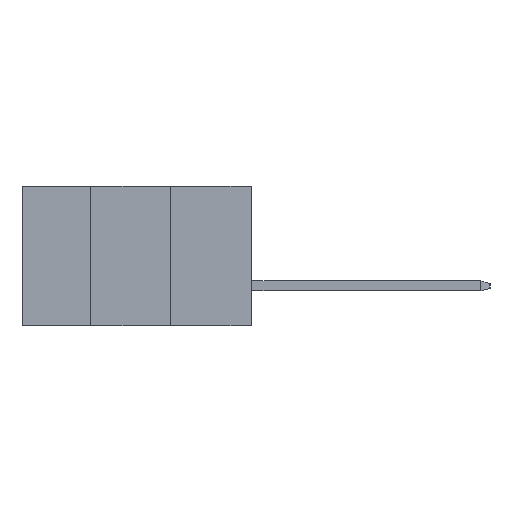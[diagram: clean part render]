
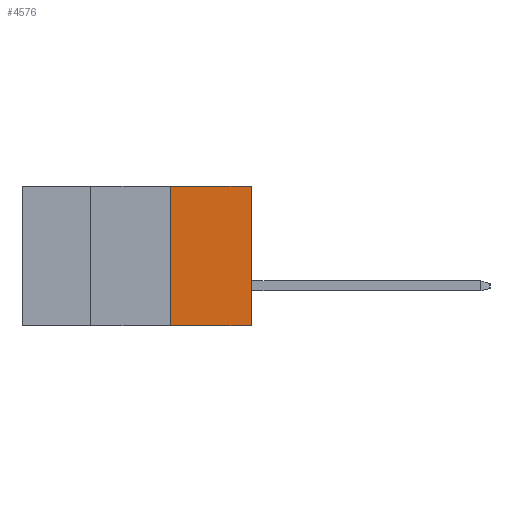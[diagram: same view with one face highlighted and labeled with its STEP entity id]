
A CAD part, left-side view. The second image highlights one B-rep face of the part: STEP entity #4576.
In plain terms, the highlighted planar face has unit normal (-1, 0, 0).
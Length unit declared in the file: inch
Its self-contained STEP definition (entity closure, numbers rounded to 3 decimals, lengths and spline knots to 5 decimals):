
#219 = CARTESIAN_POINT ( 'NONE',  ( 0.4265, 0.254, -0.437 ) ) ;
#286 = FACE_OUTER_BOUND ( 'NONE', #6150, .T. ) ;
#688 = ORIENTED_EDGE ( 'NONE', *, *, #4879, .F. ) ;
#712 = CARTESIAN_POINT ( 'NONE',  ( 0.4265, 0.254, -0.437 ) ) ;
#880 = DIRECTION ( 'NONE',  ( 0., 0., 1. ) ) ;
#1034 = CARTESIAN_POINT ( 'NONE',  ( 0.4265, 0.254, 0. ) ) ;
#1666 = LINE ( 'NONE', #712, #5442 ) ;
#2535 = EDGE_CURVE ( 'NONE', #9106, #3248, #8059, .T. ) ;
#2628 = DIRECTION ( 'NONE',  ( 0., -1., 0. ) ) ;
#3248 = VERTEX_POINT ( 'NONE', #3472 ) ;
#3455 = ORIENTED_EDGE ( 'NONE', *, *, #5671, .T. ) ;
#3472 = CARTESIAN_POINT ( 'NONE',  ( 0.4265, 0., 0. ) ) ;
#3785 = ORIENTED_EDGE ( 'NONE', *, *, #2535, .F. ) ;
#3966 = AXIS2_PLACEMENT_3D ( 'NONE', #219, #9567, #7737 ) ;
#4004 = PLANE ( 'NONE',  #3966 ) ;
#4518 = CARTESIAN_POINT ( 'NONE',  ( 0.4265, 0.254, -0.437 ) ) ;
#4576 = ADVANCED_FACE ( 'NONE', ( #286 ), #4004, .F. ) ;
#4879 = EDGE_CURVE ( 'NONE', #10800, #9106, #1666, .T. ) ;
#4969 = EDGE_CURVE ( 'NONE', #7270, #3248, #7228, .T. ) ;
#5320 = DIRECTION ( 'NONE',  ( 0., 0., 1. ) ) ;
#5442 = VECTOR ( 'NONE', #5320, 39.37008 ) ;
#5671 = EDGE_CURVE ( 'NONE', #10800, #7270, #8198, .T. ) ;
#6150 = EDGE_LOOP ( 'NONE', ( #8887, #3785, #688, #3455 ) ) ;
#6300 = VECTOR ( 'NONE', #2628, 39.37008 ) ;
#6307 = CARTESIAN_POINT ( 'NONE',  ( 0.4265, 0., -0.437 ) ) ;
#6431 = VECTOR ( 'NONE', #880, 39.37008 ) ;
#7228 = LINE ( 'NONE', #6307, #6431 ) ;
#7266 = CARTESIAN_POINT ( 'NONE',  ( 0.4265, 0.254, 0. ) ) ;
#7270 = VERTEX_POINT ( 'NONE', #9512 ) ;
#7737 = DIRECTION ( 'NONE',  ( 0., 0., -1. ) ) ;
#8059 = LINE ( 'NONE', #7266, #6300 ) ;
#8198 = LINE ( 'NONE', #4518, #8853 ) ;
#8853 = VECTOR ( 'NONE', #11735, 39.37008 ) ;
#8887 = ORIENTED_EDGE ( 'NONE', *, *, #4969, .T. ) ;
#9106 = VERTEX_POINT ( 'NONE', #1034 ) ;
#9512 = CARTESIAN_POINT ( 'NONE',  ( 0.4265, 0., -0.437 ) ) ;
#9567 = DIRECTION ( 'NONE',  ( 1., 0., 0. ) ) ;
#10800 = VERTEX_POINT ( 'NONE', #11706 ) ;
#11706 = CARTESIAN_POINT ( 'NONE',  ( 0.4265, 0.254, -0.437 ) ) ;
#11735 = DIRECTION ( 'NONE',  ( 0., -1., 0. ) ) ;
